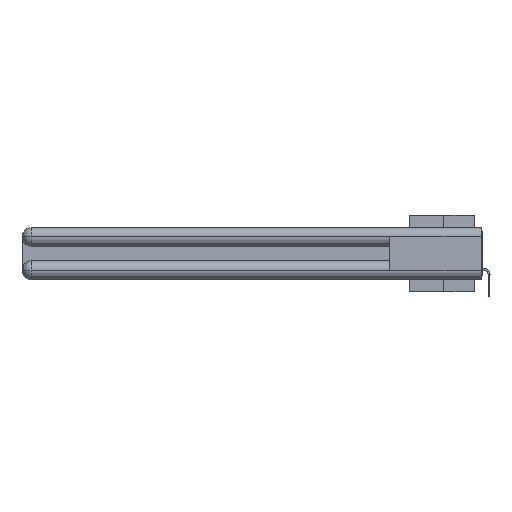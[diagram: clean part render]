
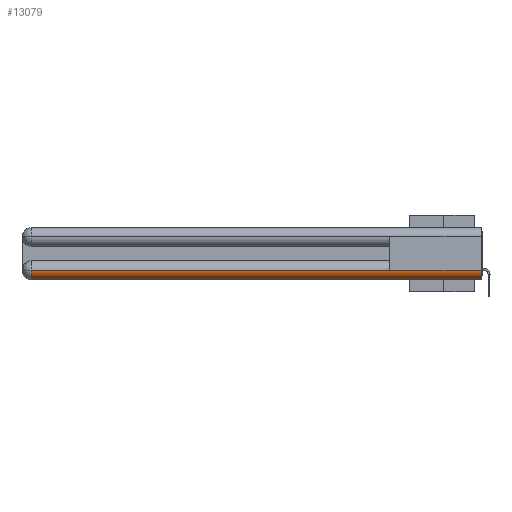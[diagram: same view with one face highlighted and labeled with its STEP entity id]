
A CAD part, left-side view. The second image highlights one B-rep face of the part: STEP entity #13079.
In plain terms, the highlighted cylindrical face has radius 1.562 mm (diameter 3.124 mm), a partial arc.
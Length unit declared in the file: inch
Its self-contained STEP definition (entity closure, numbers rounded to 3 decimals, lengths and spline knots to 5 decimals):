
#869 = CARTESIAN_POINT ( 'NONE',  ( 0., 0., -0.2785 ) ) ;
#1390 = LINE ( 'NONE', #33182, #25027 ) ;
#1885 = EDGE_CURVE ( 'NONE', #27617, #28047, #33558, .T. ) ;
#2452 = DIRECTION ( 'NONE',  ( 0., 1., 0. ) ) ;
#3296 = DIRECTION ( 'NONE',  ( 0., -1., 0. ) ) ;
#3465 = AXIS2_PLACEMENT_3D ( 'NONE', #19190, #21728, #31992 ) ;
#4464 = EDGE_CURVE ( 'NONE', #7606, #27617, #23272, .T. ) ;
#4935 = CARTESIAN_POINT ( 'NONE',  ( 0.0615, 0., -0.34 ) ) ;
#5672 = VERTEX_POINT ( 'NONE', #8407 ) ;
#7606 = VERTEX_POINT ( 'NONE', #22484 ) ;
#8407 = CARTESIAN_POINT ( 'NONE',  ( 0.0615, 2.94, -0.34 ) ) ;
#8589 = CARTESIAN_POINT ( 'NONE',  ( 0., 0., -0.2785 ) ) ;
#8939 = DIRECTION ( 'NONE',  ( 0., 1., 0. ) ) ;
#9980 = EDGE_LOOP ( 'NONE', ( #12545, #28153, #16812, #24309, #28753 ) ) ;
#11170 = AXIS2_PLACEMENT_3D ( 'NONE', #27007, #3296, #22475 ) ;
#11950 = VECTOR ( 'NONE', #2452, 39.37008 ) ;
#12187 = DIRECTION ( 'NONE',  ( 0., -1., 0. ) ) ;
#12503 = VERTEX_POINT ( 'NONE', #28526 ) ;
#12545 = ORIENTED_EDGE ( 'NONE', *, *, #20694, .T. ) ;
#13021 = CIRCLE ( 'NONE', #3465, 0.0615 ) ;
#13079 = ADVANCED_FACE ( 'NONE', ( #34271 ), #18418, .T. ) ;
#14240 = DIRECTION ( 'NONE',  ( 1., 0., 0. ) ) ;
#16430 = LINE ( 'NONE', #29436, #11950 ) ;
#16812 = ORIENTED_EDGE ( 'NONE', *, *, #25975, .F. ) ;
#18418 = CYLINDRICAL_SURFACE ( 'NONE', #11170, 0.0615 ) ;
#19190 = CARTESIAN_POINT ( 'NONE',  ( 0.0615, 2.94, -0.2785 ) ) ;
#20694 = EDGE_CURVE ( 'NONE', #7606, #12503, #16430, .T. ) ;
#21728 = DIRECTION ( 'NONE',  ( 0., -1., 0. ) ) ;
#22475 = DIRECTION ( 'NONE',  ( 0., 0., -1. ) ) ;
#22484 = CARTESIAN_POINT ( 'NONE',  ( 0., 0.6, -0.2785 ) ) ;
#23272 = LINE ( 'NONE', #869, #24492 ) ;
#24083 = AXIS2_PLACEMENT_3D ( 'NONE', #25396, #12187, #14240 ) ;
#24309 = ORIENTED_EDGE ( 'NONE', *, *, #1885, .F. ) ;
#24492 = VECTOR ( 'NONE', #32512, 39.37008 ) ;
#25027 = VECTOR ( 'NONE', #8939, 39.37008 ) ;
#25396 = CARTESIAN_POINT ( 'NONE',  ( 0.0615, 0., -0.2785 ) ) ;
#25975 = EDGE_CURVE ( 'NONE', #28047, #5672, #1390, .T. ) ;
#27007 = CARTESIAN_POINT ( 'NONE',  ( 0.0615, 0., -0.2785 ) ) ;
#27617 = VERTEX_POINT ( 'NONE', #8589 ) ;
#28047 = VERTEX_POINT ( 'NONE', #4935 ) ;
#28153 = ORIENTED_EDGE ( 'NONE', *, *, #32418, .T. ) ;
#28526 = CARTESIAN_POINT ( 'NONE',  ( 0., 2.94, -0.2785 ) ) ;
#28753 = ORIENTED_EDGE ( 'NONE', *, *, #4464, .F. ) ;
#29436 = CARTESIAN_POINT ( 'NONE',  ( 0., 0., -0.2785 ) ) ;
#31992 = DIRECTION ( 'NONE',  ( 0., 0., 1. ) ) ;
#32418 = EDGE_CURVE ( 'NONE', #12503, #5672, #13021, .T. ) ;
#32512 = DIRECTION ( 'NONE',  ( 0., -1., 0. ) ) ;
#33182 = CARTESIAN_POINT ( 'NONE',  ( 0.0615, 0., -0.34 ) ) ;
#33558 = CIRCLE ( 'NONE', #24083, 0.0615 ) ;
#34271 = FACE_OUTER_BOUND ( 'NONE', #9980, .T. ) ;
